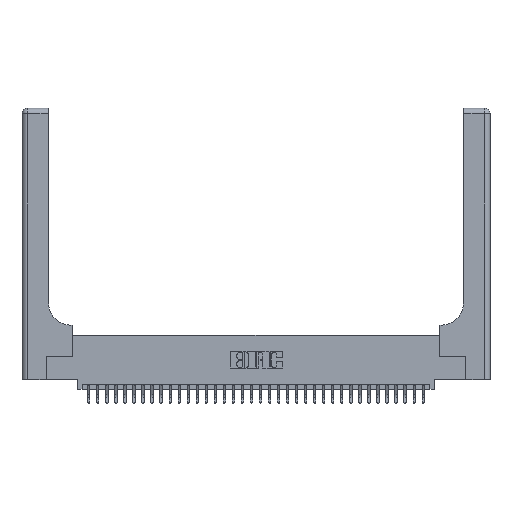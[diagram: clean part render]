
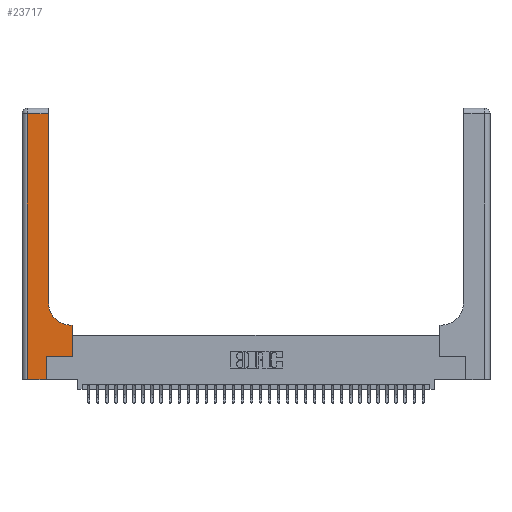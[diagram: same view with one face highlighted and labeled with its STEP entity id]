
A CAD part, top view. The second image highlights one B-rep face of the part: STEP entity #23717.
In plain terms, the highlighted planar face has unit normal (0, 0, 1).
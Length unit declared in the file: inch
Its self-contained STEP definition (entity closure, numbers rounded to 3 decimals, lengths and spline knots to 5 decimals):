
#970 = CARTESIAN_POINT ( 'NONE',  ( 0., 3., 0.37 ) ) ;
#971 = LINE ( 'NONE', #5870, #7472 ) ;
#1351 = DIRECTION ( 'NONE',  ( 0., 0., -1. ) ) ;
#1463 = PLANE ( 'NONE',  #2334 ) ;
#1606 = EDGE_CURVE ( 'NONE', #29822, #23964, #26402, .T. ) ;
#1953 = DIRECTION ( 'NONE',  ( 0., 1., 0. ) ) ;
#2130 = VERTEX_POINT ( 'NONE', #6128 ) ;
#2334 = AXIS2_PLACEMENT_3D ( 'NONE', #970, #1351, #23460 ) ;
#2405 = CARTESIAN_POINT ( 'NONE',  ( 0., 2.94, 0.37 ) ) ;
#3205 = ORIENTED_EDGE ( 'NONE', *, *, #8827, .T. ) ;
#3295 = VERTEX_POINT ( 'NONE', #26129 ) ;
#3626 = CARTESIAN_POINT ( 'NONE',  ( 0.269, 0., 0.37 ) ) ;
#3993 = ORIENTED_EDGE ( 'NONE', *, *, #5910, .T. ) ;
#4068 = VERTEX_POINT ( 'NONE', #28433 ) ;
#5003 = LINE ( 'NONE', #7663, #27513 ) ;
#5282 = VERTEX_POINT ( 'NONE', #23909 ) ;
#5542 = DIRECTION ( 'NONE',  ( 0., -1., 0. ) ) ;
#5870 = CARTESIAN_POINT ( 'NONE',  ( 0., 0., 0.37 ) ) ;
#5908 = ORIENTED_EDGE ( 'NONE', *, *, #19014, .T. ) ;
#5910 = EDGE_CURVE ( 'NONE', #4068, #2130, #12403, .T. ) ;
#6128 = CARTESIAN_POINT ( 'NONE',  ( 0.269, 0.25, 0.37 ) ) ;
#7472 = VECTOR ( 'NONE', #14543, 39.37008 ) ;
#7663 = CARTESIAN_POINT ( 'NONE',  ( 0.2915, 0.6, 0.37 ) ) ;
#8311 = VERTEX_POINT ( 'NONE', #17685 ) ;
#8827 = EDGE_CURVE ( 'NONE', #23964, #3295, #16789, .T. ) ;
#8849 = LINE ( 'NONE', #24807, #10158 ) ;
#8910 = AXIS2_PLACEMENT_3D ( 'NONE', #17775, #12423, #31654 ) ;
#9409 = VECTOR ( 'NONE', #15779, 39.37008 ) ;
#9433 = CARTESIAN_POINT ( 'NONE',  ( 0.5415, 0.6, 0.37 ) ) ;
#9596 = EDGE_CURVE ( 'NONE', #8311, #34394, #18935, .T. ) ;
#10158 = VECTOR ( 'NONE', #5542, 39.37008 ) ;
#10705 = EDGE_CURVE ( 'NONE', #34394, #22659, #5003, .T. ) ;
#12403 = LINE ( 'NONE', #3626, #27649 ) ;
#12423 = DIRECTION ( 'NONE',  ( 0., 0., -1. ) ) ;
#14119 = DIRECTION ( 'NONE',  ( -1., 0., 0. ) ) ;
#14543 = DIRECTION ( 'NONE',  ( 1., 0., 0. ) ) ;
#15190 = CARTESIAN_POINT ( 'NONE',  ( 0.5585, 0.6, 0.37 ) ) ;
#15779 = DIRECTION ( 'NONE',  ( -1., 0., 0. ) ) ;
#16789 = LINE ( 'NONE', #2405, #9409 ) ;
#17517 = EDGE_CURVE ( 'NONE', #5282, #4068, #971, .T. ) ;
#17678 = CIRCLE ( 'NONE', #8910, 0.25 ) ;
#17685 = CARTESIAN_POINT ( 'NONE',  ( 0.5585, 0.25, 0.37 ) ) ;
#17775 = CARTESIAN_POINT ( 'NONE',  ( 0.5415, 0.85, 0.37 ) ) ;
#18935 = LINE ( 'NONE', #34179, #24993 ) ;
#19014 = EDGE_CURVE ( 'NONE', #2130, #8311, #26400, .T. ) ;
#20032 = CARTESIAN_POINT ( 'NONE',  ( 0.269, 0.25, 0.37 ) ) ;
#21384 = EDGE_CURVE ( 'NONE', #22659, #29822, #17678, .T. ) ;
#22659 = VERTEX_POINT ( 'NONE', #9433 ) ;
#23460 = DIRECTION ( 'NONE',  ( -1., 0., 0. ) ) ;
#23717 = ADVANCED_FACE ( 'NONE', ( #26721 ), #1463, .F. ) ;
#23818 = CARTESIAN_POINT ( 'NONE',  ( 0.2915, 2.94, 0.37 ) ) ;
#23909 = CARTESIAN_POINT ( 'NONE',  ( 0.06, 0., 0.37 ) ) ;
#23964 = VERTEX_POINT ( 'NONE', #23818 ) ;
#24327 = CARTESIAN_POINT ( 'NONE',  ( 0.2915, 3., 0.37 ) ) ;
#24711 = ORIENTED_EDGE ( 'NONE', *, *, #9596, .T. ) ;
#24807 = CARTESIAN_POINT ( 'NONE',  ( 0.06, 3., 0.37 ) ) ;
#24993 = VECTOR ( 'NONE', #28671, 39.37008 ) ;
#26129 = CARTESIAN_POINT ( 'NONE',  ( 0.06, 2.94, 0.37 ) ) ;
#26400 = LINE ( 'NONE', #20032, #32564 ) ;
#26402 = LINE ( 'NONE', #24327, #32528 ) ;
#26679 = ORIENTED_EDGE ( 'NONE', *, *, #21384, .T. ) ;
#26721 = FACE_OUTER_BOUND ( 'NONE', #33655, .T. ) ;
#27406 = ORIENTED_EDGE ( 'NONE', *, *, #10705, .T. ) ;
#27513 = VECTOR ( 'NONE', #14119, 39.37008 ) ;
#27649 = VECTOR ( 'NONE', #34433, 39.37008 ) ;
#28317 = DIRECTION ( 'NONE',  ( 1., 0., 0. ) ) ;
#28433 = CARTESIAN_POINT ( 'NONE',  ( 0.269, 0., 0.37 ) ) ;
#28671 = DIRECTION ( 'NONE',  ( 0., 1., 0. ) ) ;
#29651 = ORIENTED_EDGE ( 'NONE', *, *, #29986, .T. ) ;
#29822 = VERTEX_POINT ( 'NONE', #30299 ) ;
#29986 = EDGE_CURVE ( 'NONE', #3295, #5282, #8849, .T. ) ;
#30299 = CARTESIAN_POINT ( 'NONE',  ( 0.2915, 0.85, 0.37 ) ) ;
#31654 = DIRECTION ( 'NONE',  ( 1., 0., 0. ) ) ;
#32528 = VECTOR ( 'NONE', #1953, 39.37008 ) ;
#32564 = VECTOR ( 'NONE', #28317, 39.37008 ) ;
#33655 = EDGE_LOOP ( 'NONE', ( #33968, #3205, #29651, #35900, #3993, #5908, #24711, #27406, #26679 ) ) ;
#33968 = ORIENTED_EDGE ( 'NONE', *, *, #1606, .T. ) ;
#34179 = CARTESIAN_POINT ( 'NONE',  ( 0.5585, 0.25, 0.37 ) ) ;
#34394 = VERTEX_POINT ( 'NONE', #15190 ) ;
#34433 = DIRECTION ( 'NONE',  ( 0., 1., 0. ) ) ;
#35900 = ORIENTED_EDGE ( 'NONE', *, *, #17517, .T. ) ;
